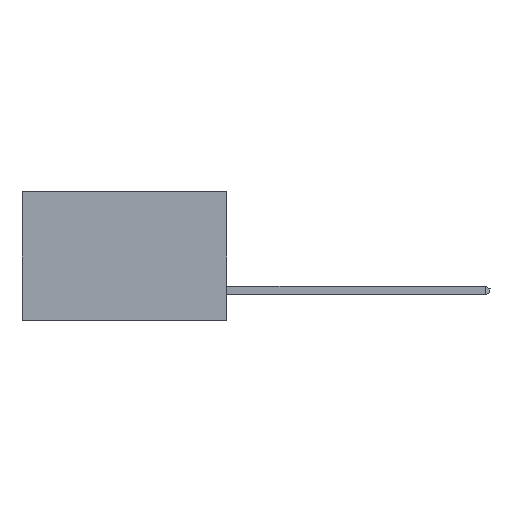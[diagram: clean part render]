
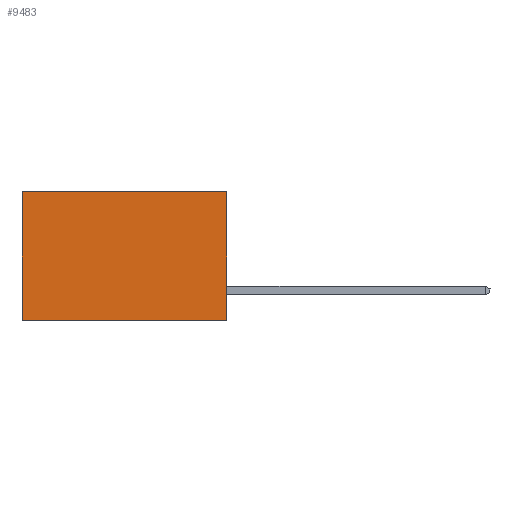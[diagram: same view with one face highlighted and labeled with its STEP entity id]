
A CAD part, left-side view. The second image highlights one B-rep face of the part: STEP entity #9483.
In plain terms, the highlighted planar face has unit normal (-1, 0, 0).
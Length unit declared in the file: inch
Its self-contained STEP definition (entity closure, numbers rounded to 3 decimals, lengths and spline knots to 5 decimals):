
#584 = LINE ( 'NONE', #11466, #11871 ) ;
#1152 = VERTEX_POINT ( 'NONE', #8723 ) ;
#1343 = CARTESIAN_POINT ( 'NONE',  ( 0.277, 0.59, -0.37 ) ) ;
#2477 = DIRECTION ( 'NONE',  ( 0., 0., -1. ) ) ;
#2508 = DIRECTION ( 'NONE',  ( 1., 0., 0. ) ) ;
#2561 = CARTESIAN_POINT ( 'NONE',  ( 0.277, 0., -0.37 ) ) ;
#2574 = PLANE ( 'NONE',  #9923 ) ;
#2997 = VERTEX_POINT ( 'NONE', #8374 ) ;
#3420 = CARTESIAN_POINT ( 'NONE',  ( 0.277, 0., 0. ) ) ;
#3583 = EDGE_LOOP ( 'NONE', ( #12192, #9560, #12539, #6914 ) ) ;
#3649 = DIRECTION ( 'NONE',  ( 0., 0., -1. ) ) ;
#3891 = VERTEX_POINT ( 'NONE', #14285 ) ;
#4265 = DIRECTION ( 'NONE',  ( 0., 1., 0. ) ) ;
#4491 = LINE ( 'NONE', #5046, #9716 ) ;
#4757 = VECTOR ( 'NONE', #3649, 39.37008 ) ;
#5046 = CARTESIAN_POINT ( 'NONE',  ( 0.277, 0., -0.37 ) ) ;
#5121 = DIRECTION ( 'NONE',  ( 0., 1., 0. ) ) ;
#6503 = EDGE_CURVE ( 'NONE', #13665, #3891, #584, .T. ) ;
#6914 = ORIENTED_EDGE ( 'NONE', *, *, #11732, .T. ) ;
#7499 = EDGE_CURVE ( 'NONE', #3891, #1152, #4491, .T. ) ;
#8374 = CARTESIAN_POINT ( 'NONE',  ( 0.277, 0.59, 0. ) ) ;
#8557 = VECTOR ( 'NONE', #4265, 39.37008 ) ;
#8723 = CARTESIAN_POINT ( 'NONE',  ( 0.277, 0.59, -0.37 ) ) ;
#9483 = ADVANCED_FACE ( 'NONE', ( #10026 ), #2574, .F. ) ;
#9560 = ORIENTED_EDGE ( 'NONE', *, *, #7499, .F. ) ;
#9716 = VECTOR ( 'NONE', #5121, 39.37008 ) ;
#9821 = CARTESIAN_POINT ( 'NONE',  ( 0.277, 0., 0. ) ) ;
#9923 = AXIS2_PLACEMENT_3D ( 'NONE', #2561, #2508, #2477 ) ;
#10026 = FACE_OUTER_BOUND ( 'NONE', #3583, .T. ) ;
#10654 = EDGE_CURVE ( 'NONE', #2997, #1152, #13593, .T. ) ;
#11466 = CARTESIAN_POINT ( 'NONE',  ( 0.277, 0., -0.37 ) ) ;
#11578 = LINE ( 'NONE', #9821, #8557 ) ;
#11732 = EDGE_CURVE ( 'NONE', #13665, #2997, #11578, .T. ) ;
#11871 = VECTOR ( 'NONE', #13668, 39.37008 ) ;
#12192 = ORIENTED_EDGE ( 'NONE', *, *, #10654, .T. ) ;
#12539 = ORIENTED_EDGE ( 'NONE', *, *, #6503, .F. ) ;
#13593 = LINE ( 'NONE', #1343, #4757 ) ;
#13665 = VERTEX_POINT ( 'NONE', #3420 ) ;
#13668 = DIRECTION ( 'NONE',  ( 0., 0., -1. ) ) ;
#14285 = CARTESIAN_POINT ( 'NONE',  ( 0.277, 0., -0.37 ) ) ;
